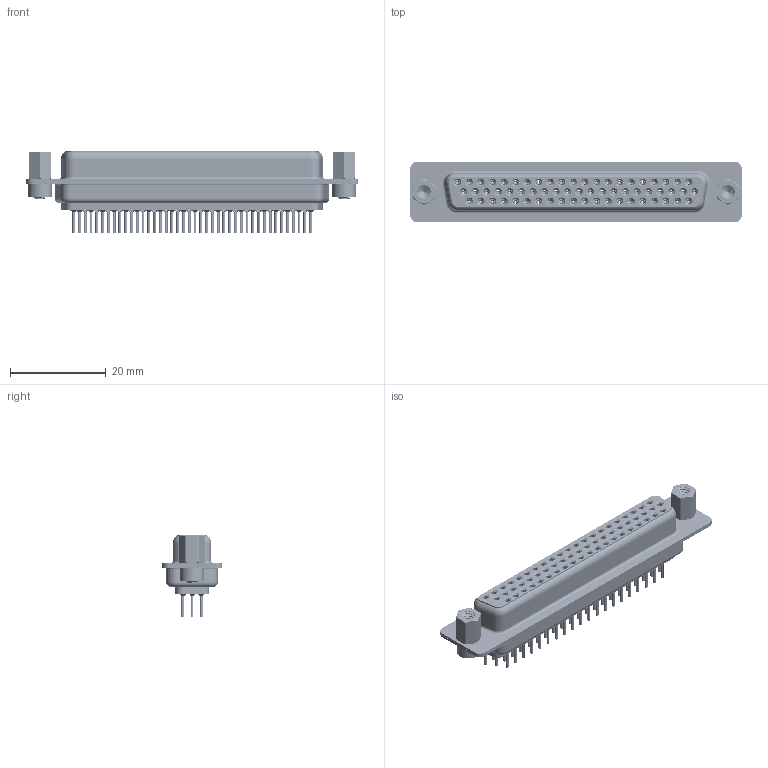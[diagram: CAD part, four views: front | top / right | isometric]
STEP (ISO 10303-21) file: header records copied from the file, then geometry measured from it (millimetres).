
FILE_DESCRIPTION (( 'STEP AP203' ), '1' );
FILE_NAME ('638-062-330-243.STEP', '2020-07-19T01:43:29', ( '' ), ( '' ), 'SwSTEP 2.0', 'SolidWorks 2020', '' );
FILE_SCHEMA (( 'CONFIG_CONTROL_DESIGN' ));
Length unit declared in the file: millimetre
Products named in the file (9): 638 Contact Row 2_30; 638 4-40 Threaded Rivet; 638-062-330-243; 638 Shell Front_62 Contacts; 638 Contact Row 3_30; 638 Shell Rear_62 Contacts; 638 Housing_62 Contacts; 638 Contact Row 1_30; 638 4-40 Hex Standoff
Assembly tree (69 placements, depth 2):
  638-062-330-243
    638 Housing_62 Contacts
    638 Shell Front_62 Contacts
    638 Shell Rear_62 Contacts
    638 Contact Row 1_30  x21
    638 Contact Row 2_30  x21
    638 Contact Row 3_30  x20
    638 4-40 Threaded Rivet  x2
    638 4-40 Hex Standoff  x2
Bounding box: 69.32 x 12.6 x 17.3 mm (x, y, z)
Volume: 4809.5 mm3; surface area: 17945.3 mm2
Topology: 69 solids, 69 shells, 8279 faces, 21121 edges, 13115 vertices
Faces by surface type: cylinder 2255, plane 2011, torus 1669, bspline 1258, cone 1086
Entity records: 51766 total; most frequent: CARTESIAN_POINT 15154, DIRECTION 7571, ORIENTED_EDGE 6770, EDGE_CURVE 3385, AXIS2_PLACEMENT_3D 3197, VERTEX_POINT 2147, EDGE_LOOP 1786, CIRCLE 1743
